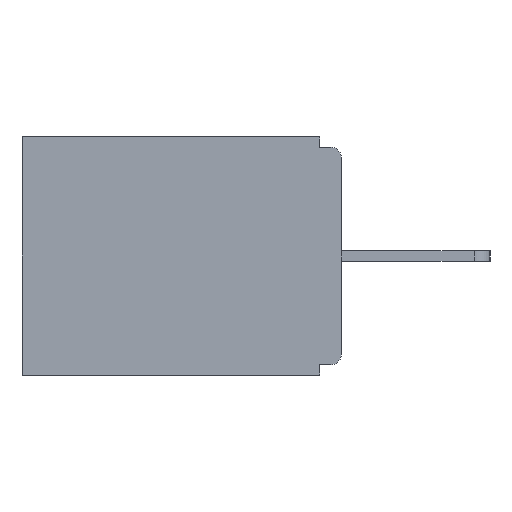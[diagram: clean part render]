
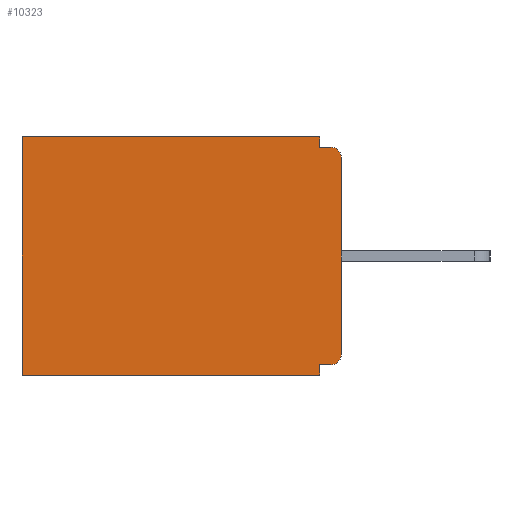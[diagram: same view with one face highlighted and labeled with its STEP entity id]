
A CAD part, left-side view. The second image highlights one B-rep face of the part: STEP entity #10323.
In plain terms, the highlighted planar face has unit normal (-1, 0, 0).
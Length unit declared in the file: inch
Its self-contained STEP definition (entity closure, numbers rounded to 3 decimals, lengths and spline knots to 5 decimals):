
#163 = CARTESIAN_POINT ( 'NONE',  ( 0.298, 0.015, -0.03 ) ) ;
#271 = LINE ( 'NONE', #12692, #8525 ) ;
#830 = EDGE_CURVE ( 'NONE', #8735, #14389, #867, .T. ) ;
#867 = LINE ( 'NONE', #945, #14259 ) ;
#887 = CARTESIAN_POINT ( 'NONE',  ( 0.298, 0.015, -0.015 ) ) ;
#945 = CARTESIAN_POINT ( 'NONE',  ( 0.298, 0., 0. ) ) ;
#1534 = VERTEX_POINT ( 'NONE', #7921 ) ;
#1668 = AXIS2_PLACEMENT_3D ( 'NONE', #9741, #13713, #2453 ) ;
#1699 = VERTEX_POINT ( 'NONE', #10700 ) ;
#1731 = DIRECTION ( 'NONE',  ( -1., 0., 0. ) ) ;
#1795 = ORIENTED_EDGE ( 'NONE', *, *, #830, .F. ) ;
#1814 = CARTESIAN_POINT ( 'NONE',  ( 0.298, 0.031, -0.015 ) ) ;
#2009 = VECTOR ( 'NONE', #16174, 39.37008 ) ;
#2085 = LINE ( 'NONE', #13195, #14452 ) ;
#2094 = CARTESIAN_POINT ( 'NONE',  ( 0.298, 0., -0.03 ) ) ;
#2134 = EDGE_CURVE ( 'NONE', #15484, #1534, #13523, .T. ) ;
#2453 = DIRECTION ( 'NONE',  ( 0., 0., -1. ) ) ;
#2717 = EDGE_CURVE ( 'NONE', #4483, #6847, #15555, .T. ) ;
#2894 = DIRECTION ( 'NONE',  ( 0., 1., 0. ) ) ;
#2976 = ORIENTED_EDGE ( 'NONE', *, *, #2717, .T. ) ;
#3297 = ORIENTED_EDGE ( 'NONE', *, *, #11588, .T. ) ;
#3617 = LINE ( 'NONE', #8680, #12184 ) ;
#3665 = DIRECTION ( 'NONE',  ( 0., 0., -1. ) ) ;
#3701 = ORIENTED_EDGE ( 'NONE', *, *, #16130, .F. ) ;
#3997 = ORIENTED_EDGE ( 'NONE', *, *, #12183, .F. ) ;
#4483 = VERTEX_POINT ( 'NONE', #12672 ) ;
#4508 = PLANE ( 'NONE',  #1668 ) ;
#5061 = ORIENTED_EDGE ( 'NONE', *, *, #12715, .T. ) ;
#5287 = DIRECTION ( 'NONE',  ( 0., 0., -1. ) ) ;
#5722 = LINE ( 'NONE', #10775, #13797 ) ;
#5768 = FACE_OUTER_BOUND ( 'NONE', #12384, .T. ) ;
#5819 = DIRECTION ( 'NONE',  ( 0., 0., -1. ) ) ;
#5907 = CIRCLE ( 'NONE', #13302, 0.015 ) ;
#6030 = CARTESIAN_POINT ( 'NONE',  ( 0.298, 0.031, -0.328 ) ) ;
#6206 = EDGE_CURVE ( 'NONE', #6460, #10823, #3617, .T. ) ;
#6460 = VERTEX_POINT ( 'NONE', #1814 ) ;
#6625 = CARTESIAN_POINT ( 'NONE',  ( 0.298, 0.46, 0. ) ) ;
#6847 = VERTEX_POINT ( 'NONE', #10739 ) ;
#6870 = ORIENTED_EDGE ( 'NONE', *, *, #13903, .F. ) ;
#7186 = CARTESIAN_POINT ( 'NONE',  ( 0.298, 0.015, -0.313 ) ) ;
#7329 = CARTESIAN_POINT ( 'NONE',  ( 0.298, 0.015, -0.328 ) ) ;
#7916 = CARTESIAN_POINT ( 'NONE',  ( 0.298, 0., -0.313 ) ) ;
#7921 = CARTESIAN_POINT ( 'NONE',  ( 0.298, 0.031, -0.343 ) ) ;
#8525 = VECTOR ( 'NONE', #8787, 39.37008 ) ;
#8680 = CARTESIAN_POINT ( 'NONE',  ( 0.298, 0., -0.015 ) ) ;
#8735 = VERTEX_POINT ( 'NONE', #2094 ) ;
#8787 = DIRECTION ( 'NONE',  ( 0., 1., 0. ) ) ;
#9138 = DIRECTION ( 'NONE',  ( 0., 1., 0. ) ) ;
#9235 = EDGE_CURVE ( 'NONE', #8735, #10823, #10053, .T. ) ;
#9741 = CARTESIAN_POINT ( 'NONE',  ( 0.298, 0., 0. ) ) ;
#9868 = DIRECTION ( 'NONE',  ( 0., 0., -1. ) ) ;
#10053 = CIRCLE ( 'NONE', #12717, 0.015 ) ;
#10189 = DIRECTION ( 'NONE',  ( 0., -1., 0. ) ) ;
#10303 = CARTESIAN_POINT ( 'NONE',  ( 0.298, 0., -0.328 ) ) ;
#10323 = ADVANCED_FACE ( 'NONE', ( #5768 ), #4508, .F. ) ;
#10700 = CARTESIAN_POINT ( 'NONE',  ( 0.298, 0.031, 0. ) ) ;
#10739 = CARTESIAN_POINT ( 'NONE',  ( 0.298, 0.46, -0.343 ) ) ;
#10775 = CARTESIAN_POINT ( 'NONE',  ( 0.298, 0., 0. ) ) ;
#10823 = VERTEX_POINT ( 'NONE', #887 ) ;
#11588 = EDGE_CURVE ( 'NONE', #12051, #14389, #5907, .T. ) ;
#11642 = LINE ( 'NONE', #10303, #14562 ) ;
#11835 = ORIENTED_EDGE ( 'NONE', *, *, #9235, .T. ) ;
#12051 = VERTEX_POINT ( 'NONE', #7329 ) ;
#12183 = EDGE_CURVE ( 'NONE', #12051, #15484, #11642, .T. ) ;
#12184 = VECTOR ( 'NONE', #10189, 39.37008 ) ;
#12384 = EDGE_LOOP ( 'NONE', ( #11835, #14425, #3701, #5061, #2976, #6870, #13381, #3997, #3297, #1795 ) ) ;
#12672 = CARTESIAN_POINT ( 'NONE',  ( 0.298, 0.46, 0. ) ) ;
#12692 = CARTESIAN_POINT ( 'NONE',  ( 0.298, 0., -0.343 ) ) ;
#12715 = EDGE_CURVE ( 'NONE', #1699, #4483, #5722, .T. ) ;
#12717 = AXIS2_PLACEMENT_3D ( 'NONE', #163, #1731, #12751 ) ;
#12751 = DIRECTION ( 'NONE',  ( 0., 0., -1. ) ) ;
#12872 = VECTOR ( 'NONE', #5287, 39.37008 ) ;
#13195 = CARTESIAN_POINT ( 'NONE',  ( 0.298, 0.031, -0.343 ) ) ;
#13302 = AXIS2_PLACEMENT_3D ( 'NONE', #7186, #16047, #3665 ) ;
#13381 = ORIENTED_EDGE ( 'NONE', *, *, #2134, .F. ) ;
#13523 = LINE ( 'NONE', #16092, #2009 ) ;
#13713 = DIRECTION ( 'NONE',  ( 1., 0., 0. ) ) ;
#13797 = VECTOR ( 'NONE', #2894, 39.37008 ) ;
#13903 = EDGE_CURVE ( 'NONE', #1534, #6847, #271, .T. ) ;
#14259 = VECTOR ( 'NONE', #9868, 39.37008 ) ;
#14389 = VERTEX_POINT ( 'NONE', #7916 ) ;
#14425 = ORIENTED_EDGE ( 'NONE', *, *, #6206, .F. ) ;
#14452 = VECTOR ( 'NONE', #5819, 39.37008 ) ;
#14562 = VECTOR ( 'NONE', #9138, 39.37008 ) ;
#15484 = VERTEX_POINT ( 'NONE', #6030 ) ;
#15555 = LINE ( 'NONE', #6625, #12872 ) ;
#16047 = DIRECTION ( 'NONE',  ( -1., 0., 0. ) ) ;
#16092 = CARTESIAN_POINT ( 'NONE',  ( 0.298, 0.031, -0.343 ) ) ;
#16130 = EDGE_CURVE ( 'NONE', #1699, #6460, #2085, .T. ) ;
#16174 = DIRECTION ( 'NONE',  ( 0., 0., -1. ) ) ;
